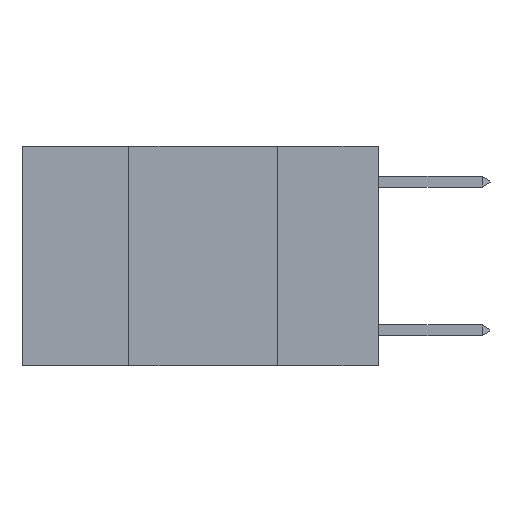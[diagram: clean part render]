
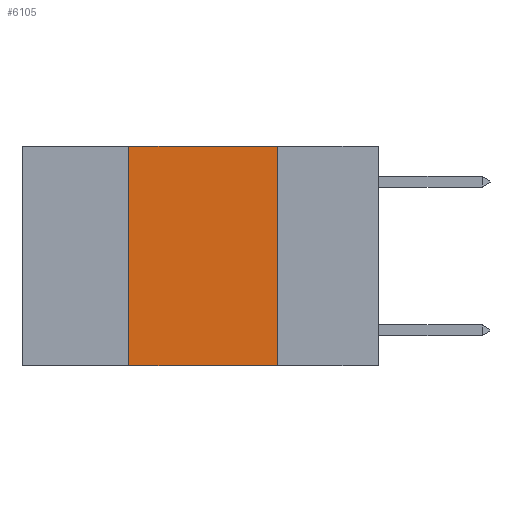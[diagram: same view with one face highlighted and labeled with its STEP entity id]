
A CAD part, left-side view. The second image highlights one B-rep face of the part: STEP entity #6105.
In plain terms, the highlighted planar face has unit normal (-1, 0, 0).
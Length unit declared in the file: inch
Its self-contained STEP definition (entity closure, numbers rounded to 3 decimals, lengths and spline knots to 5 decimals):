
#705 = EDGE_CURVE ( 'NONE', #13094, #8069, #971, .T. ) ;
#971 = LINE ( 'NONE', #6231, #1908 ) ;
#1468 = CARTESIAN_POINT ( 'NONE',  ( 0., 0.17, 0. ) ) ;
#1777 = ORIENTED_EDGE ( 'NONE', *, *, #14199, .F. ) ;
#1908 = VECTOR ( 'NONE', #12164, 39.37008 ) ;
#1948 = VECTOR ( 'NONE', #9795, 39.37008 ) ;
#3696 = PLANE ( 'NONE',  #14968 ) ;
#3850 = DIRECTION ( 'NONE',  ( 0., 0., -1. ) ) ;
#3998 = CARTESIAN_POINT ( 'NONE',  ( 0., 0.6, 0. ) ) ;
#4349 = VERTEX_POINT ( 'NONE', #14032 ) ;
#4576 = EDGE_CURVE ( 'NONE', #4349, #12628, #13001, .T. ) ;
#4614 = ORIENTED_EDGE ( 'NONE', *, *, #8825, .F. ) ;
#5156 = FACE_OUTER_BOUND ( 'NONE', #14436, .T. ) ;
#6105 = ADVANCED_FACE ( 'NONE', ( #5156 ), #3696, .F. ) ;
#6169 = DIRECTION ( 'NONE',  ( 1., 0., 0. ) ) ;
#6231 = CARTESIAN_POINT ( 'NONE',  ( 0., 0.6, 0. ) ) ;
#6294 = CARTESIAN_POINT ( 'NONE',  ( 0., 0.42, 0. ) ) ;
#6699 = ORIENTED_EDGE ( 'NONE', *, *, #705, .F. ) ;
#7233 = CARTESIAN_POINT ( 'NONE',  ( 0., 0.6, -0.37 ) ) ;
#7308 = LINE ( 'NONE', #6294, #1948 ) ;
#8069 = VERTEX_POINT ( 'NONE', #1468 ) ;
#8825 = EDGE_CURVE ( 'NONE', #4349, #13094, #7308, .T. ) ;
#9115 = CARTESIAN_POINT ( 'NONE',  ( 0., 0.17, -0.37 ) ) ;
#9480 = CARTESIAN_POINT ( 'NONE',  ( 0., 0.17, 0. ) ) ;
#9795 = DIRECTION ( 'NONE',  ( 0., 0., 1. ) ) ;
#10624 = DIRECTION ( 'NONE',  ( 0., -1., 0. ) ) ;
#11535 = ORIENTED_EDGE ( 'NONE', *, *, #4576, .T. ) ;
#12164 = DIRECTION ( 'NONE',  ( 0., -1., 0. ) ) ;
#12231 = VECTOR ( 'NONE', #10624, 39.37008 ) ;
#12628 = VERTEX_POINT ( 'NONE', #9115 ) ;
#13001 = LINE ( 'NONE', #7233, #12231 ) ;
#13094 = VERTEX_POINT ( 'NONE', #14940 ) ;
#13595 = VECTOR ( 'NONE', #14043, 39.37008 ) ;
#14032 = CARTESIAN_POINT ( 'NONE',  ( 0., 0.42, -0.37 ) ) ;
#14043 = DIRECTION ( 'NONE',  ( 0., 0., -1. ) ) ;
#14199 = EDGE_CURVE ( 'NONE', #8069, #12628, #15141, .T. ) ;
#14436 = EDGE_LOOP ( 'NONE', ( #1777, #6699, #4614, #11535 ) ) ;
#14940 = CARTESIAN_POINT ( 'NONE',  ( 0., 0.42, 0. ) ) ;
#14968 = AXIS2_PLACEMENT_3D ( 'NONE', #3998, #6169, #3850 ) ;
#15141 = LINE ( 'NONE', #9480, #13595 ) ;
